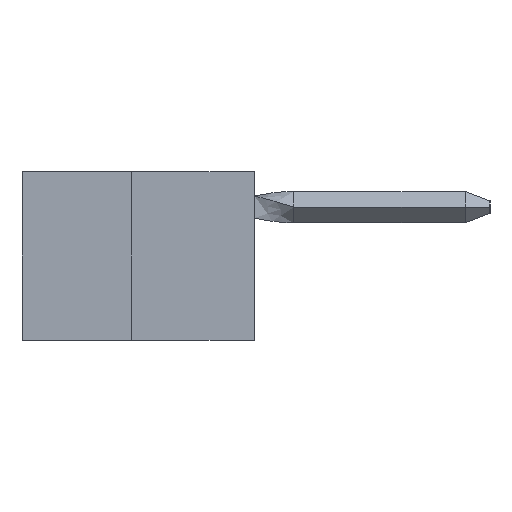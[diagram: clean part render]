
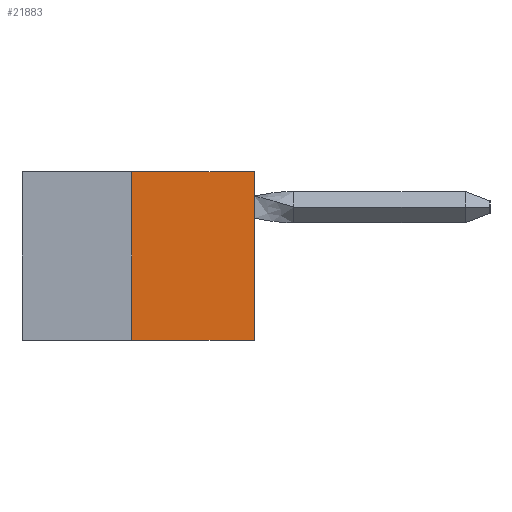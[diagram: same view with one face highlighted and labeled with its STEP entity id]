
A CAD part, left-side view. The second image highlights one B-rep face of the part: STEP entity #21883.
In plain terms, the highlighted planar face has unit normal (-1, 0, 0).
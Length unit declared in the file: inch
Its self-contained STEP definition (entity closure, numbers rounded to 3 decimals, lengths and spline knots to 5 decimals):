
#21 = DIRECTION ( 'NONE',  ( 0., -1., 0. ) ) ;
#4338 = DIRECTION ( 'NONE',  ( 0., -1., 0. ) ) ;
#4651 = CARTESIAN_POINT ( 'NONE',  ( 0., 0., -0.343 ) ) ;
#7350 = DIRECTION ( 'NONE',  ( 0., 0., -1. ) ) ;
#7726 = VERTEX_POINT ( 'NONE', #24438 ) ;
#9084 = EDGE_CURVE ( 'NONE', #20842, #36190, #36099, .T. ) ;
#9663 = CARTESIAN_POINT ( 'NONE',  ( 0., 0., 0. ) ) ;
#11485 = EDGE_CURVE ( 'NONE', #36722, #7726, #22708, .T. ) ;
#13380 = CARTESIAN_POINT ( 'NONE',  ( 0., 0.473, 0. ) ) ;
#13581 = DIRECTION ( 'NONE',  ( 1., 0., 0. ) ) ;
#14115 = EDGE_LOOP ( 'NONE', ( #36384, #29699, #18901, #23940 ) ) ;
#18301 = VECTOR ( 'NONE', #20092, 39.37008 ) ;
#18780 = LINE ( 'NONE', #28856, #18301 ) ;
#18901 = ORIENTED_EDGE ( 'NONE', *, *, #9084, .T. ) ;
#18952 = LINE ( 'NONE', #9663, #27271 ) ;
#19887 = EDGE_CURVE ( 'NONE', #20842, #36722, #18780, .T. ) ;
#20048 = VECTOR ( 'NONE', #21, 39.37008 ) ;
#20092 = DIRECTION ( 'NONE',  ( 0., 0., 1. ) ) ;
#20842 = VERTEX_POINT ( 'NONE', #36054 ) ;
#21834 = DIRECTION ( 'NONE',  ( 0., 0., 1. ) ) ;
#21883 = ADVANCED_FACE ( 'NONE', ( #36867 ), #25186, .F. ) ;
#22708 = LINE ( 'NONE', #13380, #36935 ) ;
#23940 = ORIENTED_EDGE ( 'NONE', *, *, #24018, .T. ) ;
#24018 = EDGE_CURVE ( 'NONE', #36190, #7726, #18952, .T. ) ;
#24438 = CARTESIAN_POINT ( 'NONE',  ( 0., 0., 0. ) ) ;
#25186 = PLANE ( 'NONE',  #33234 ) ;
#27271 = VECTOR ( 'NONE', #21834, 39.37008 ) ;
#28856 = CARTESIAN_POINT ( 'NONE',  ( 0., 0.25, 0. ) ) ;
#29699 = ORIENTED_EDGE ( 'NONE', *, *, #19887, .F. ) ;
#32780 = CARTESIAN_POINT ( 'NONE',  ( 0., 0.473, -0.343 ) ) ;
#33210 = CARTESIAN_POINT ( 'NONE',  ( 0., 0.25, 0. ) ) ;
#33234 = AXIS2_PLACEMENT_3D ( 'NONE', #34281, #13581, #7350 ) ;
#34281 = CARTESIAN_POINT ( 'NONE',  ( 0., 0.473, 0. ) ) ;
#36054 = CARTESIAN_POINT ( 'NONE',  ( 0., 0.25, -0.343 ) ) ;
#36099 = LINE ( 'NONE', #32780, #20048 ) ;
#36190 = VERTEX_POINT ( 'NONE', #4651 ) ;
#36384 = ORIENTED_EDGE ( 'NONE', *, *, #11485, .F. ) ;
#36722 = VERTEX_POINT ( 'NONE', #33210 ) ;
#36867 = FACE_OUTER_BOUND ( 'NONE', #14115, .T. ) ;
#36935 = VECTOR ( 'NONE', #4338, 39.37008 ) ;
